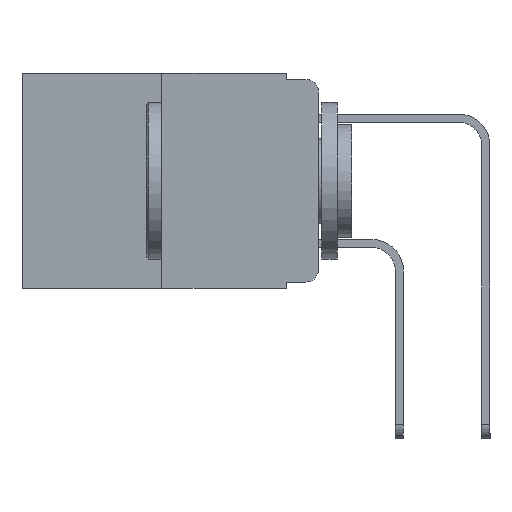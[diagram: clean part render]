
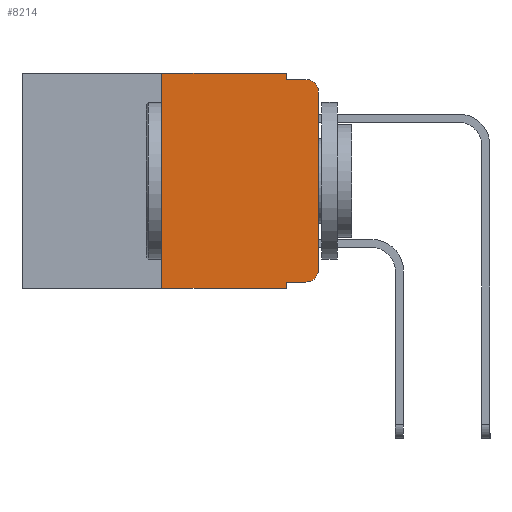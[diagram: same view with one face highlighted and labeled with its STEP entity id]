
A CAD part, left-side view. The second image highlights one B-rep face of the part: STEP entity #8214.
In plain terms, the highlighted planar face has unit normal (-1, 0, 0).
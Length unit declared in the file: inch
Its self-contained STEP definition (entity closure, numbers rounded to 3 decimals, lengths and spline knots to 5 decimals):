
#141 = CARTESIAN_POINT ( 'NONE',  ( 0., 0.473, -0.343 ) ) ;
#411 = EDGE_CURVE ( 'NONE', #4184, #6890, #11350, .T. ) ;
#431 = CARTESIAN_POINT ( 'NONE',  ( 0., 0.051, -0.333 ) ) ;
#1786 = CARTESIAN_POINT ( 'NONE',  ( 0., 0.25, 0. ) ) ;
#2180 = CARTESIAN_POINT ( 'NONE',  ( 0., 0.02, -0.333 ) ) ;
#2209 = DIRECTION ( 'NONE',  ( 0., -1., 0. ) ) ;
#2853 = AXIS2_PLACEMENT_3D ( 'NONE', #21239, #9372, #23160 ) ;
#2871 = CARTESIAN_POINT ( 'NONE',  ( 0., 0., -0.313 ) ) ;
#2944 = DIRECTION ( 'NONE',  ( 0., -1., 0. ) ) ;
#3098 = VERTEX_POINT ( 'NONE', #431 ) ;
#3100 = CARTESIAN_POINT ( 'NONE',  ( 0., 0.25, 0. ) ) ;
#3232 = VECTOR ( 'NONE', #19930, 39.37008 ) ;
#3301 = LINE ( 'NONE', #141, #13367 ) ;
#3305 = CARTESIAN_POINT ( 'NONE',  ( 0., 0.051, -0.343 ) ) ;
#3547 = CARTESIAN_POINT ( 'NONE',  ( 0., 0., -0.03 ) ) ;
#3550 = LINE ( 'NONE', #17707, #18863 ) ;
#3804 = DIRECTION ( 'NONE',  ( 0., 0., 1. ) ) ;
#4184 = VERTEX_POINT ( 'NONE', #2180 ) ;
#4240 = CARTESIAN_POINT ( 'NONE',  ( 0., 0.051, 0. ) ) ;
#4698 = EDGE_CURVE ( 'NONE', #12145, #19349, #23422, .T. ) ;
#4979 = PLANE ( 'NONE',  #25516 ) ;
#5031 = EDGE_CURVE ( 'NONE', #21617, #6190, #22497, .T. ) ;
#5187 = EDGE_CURVE ( 'NONE', #3098, #4184, #3550, .T. ) ;
#6190 = VERTEX_POINT ( 'NONE', #18696 ) ;
#6381 = EDGE_CURVE ( 'NONE', #14464, #6190, #7795, .T. ) ;
#6716 = VECTOR ( 'NONE', #2944, 39.37008 ) ;
#6890 = VERTEX_POINT ( 'NONE', #2871 ) ;
#6992 = DIRECTION ( 'NONE',  ( 0., 0., -1. ) ) ;
#7072 = FACE_OUTER_BOUND ( 'NONE', #13237, .T. ) ;
#7083 = VECTOR ( 'NONE', #19625, 39.37008 ) ;
#7795 = CIRCLE ( 'NONE', #2853, 0.02 ) ;
#8214 = ADVANCED_FACE ( 'NONE', ( #7072 ), #4979, .F. ) ;
#9088 = EDGE_CURVE ( 'NONE', #12145, #10170, #3301, .T. ) ;
#9372 = DIRECTION ( 'NONE',  ( -1., 0., 0. ) ) ;
#10170 = VERTEX_POINT ( 'NONE', #3305 ) ;
#10204 = ORIENTED_EDGE ( 'NONE', *, *, #9088, .T. ) ;
#10403 = EDGE_CURVE ( 'NONE', #6890, #14464, #13903, .T. ) ;
#11150 = AXIS2_PLACEMENT_3D ( 'NONE', #21232, #23412, #23553 ) ;
#11350 = CIRCLE ( 'NONE', #11150, 0.02 ) ;
#12002 = EDGE_CURVE ( 'NONE', #19349, #13975, #20592, .T. ) ;
#12145 = VERTEX_POINT ( 'NONE', #16692 ) ;
#12557 = ORIENTED_EDGE ( 'NONE', *, *, #10403, .T. ) ;
#13041 = VECTOR ( 'NONE', #3804, 39.37008 ) ;
#13237 = EDGE_LOOP ( 'NONE', ( #12557, #23017, #16154, #21878, #24249, #14866, #10204, #18603, #24890, #20110 ) ) ;
#13367 = VECTOR ( 'NONE', #2209, 39.37008 ) ;
#13903 = LINE ( 'NONE', #17967, #3232 ) ;
#13975 = VERTEX_POINT ( 'NONE', #20561 ) ;
#14464 = VERTEX_POINT ( 'NONE', #3547 ) ;
#14735 = VECTOR ( 'NONE', #22157, 39.37008 ) ;
#14866 = ORIENTED_EDGE ( 'NONE', *, *, #4698, .F. ) ;
#14943 = CARTESIAN_POINT ( 'NONE',  ( 0., 0.473, 0. ) ) ;
#16154 = ORIENTED_EDGE ( 'NONE', *, *, #5031, .F. ) ;
#16692 = CARTESIAN_POINT ( 'NONE',  ( 0., 0.25, -0.343 ) ) ;
#17244 = EDGE_CURVE ( 'NONE', #3098, #10170, #19143, .T. ) ;
#17673 = CARTESIAN_POINT ( 'NONE',  ( 0., 0.051, 0. ) ) ;
#17707 = CARTESIAN_POINT ( 'NONE',  ( 0., 0.051, -0.333 ) ) ;
#17967 = CARTESIAN_POINT ( 'NONE',  ( 0., 0., 0. ) ) ;
#18603 = ORIENTED_EDGE ( 'NONE', *, *, #17244, .F. ) ;
#18696 = CARTESIAN_POINT ( 'NONE',  ( 0., 0.02, -0.01 ) ) ;
#18863 = VECTOR ( 'NONE', #19659, 39.37008 ) ;
#18927 = DIRECTION ( 'NONE',  ( 1., 0., 0. ) ) ;
#19143 = LINE ( 'NONE', #4240, #23657 ) ;
#19349 = VERTEX_POINT ( 'NONE', #3100 ) ;
#19625 = DIRECTION ( 'NONE',  ( 0., 0., -1. ) ) ;
#19659 = DIRECTION ( 'NONE',  ( 0., -1., 0. ) ) ;
#19930 = DIRECTION ( 'NONE',  ( 0., 0., 1. ) ) ;
#19966 = CARTESIAN_POINT ( 'NONE',  ( 0., 0.051, -0.01 ) ) ;
#20110 = ORIENTED_EDGE ( 'NONE', *, *, #411, .T. ) ;
#20132 = CARTESIAN_POINT ( 'NONE',  ( 0., 0.473, 0. ) ) ;
#20172 = DIRECTION ( 'NONE',  ( 0., 0., -1. ) ) ;
#20561 = CARTESIAN_POINT ( 'NONE',  ( 0., 0.051, 0. ) ) ;
#20592 = LINE ( 'NONE', #20132, #14735 ) ;
#21232 = CARTESIAN_POINT ( 'NONE',  ( 0., 0.02, -0.313 ) ) ;
#21239 = CARTESIAN_POINT ( 'NONE',  ( 0., 0.02, -0.03 ) ) ;
#21491 = EDGE_CURVE ( 'NONE', #13975, #21617, #22856, .T. ) ;
#21617 = VERTEX_POINT ( 'NONE', #19966 ) ;
#21878 = ORIENTED_EDGE ( 'NONE', *, *, #21491, .F. ) ;
#22157 = DIRECTION ( 'NONE',  ( 0., -1., 0. ) ) ;
#22497 = LINE ( 'NONE', #24539, #6716 ) ;
#22856 = LINE ( 'NONE', #17673, #7083 ) ;
#23017 = ORIENTED_EDGE ( 'NONE', *, *, #6381, .T. ) ;
#23160 = DIRECTION ( 'NONE',  ( 0., 0., -1. ) ) ;
#23412 = DIRECTION ( 'NONE',  ( -1., 0., 0. ) ) ;
#23422 = LINE ( 'NONE', #1786, #13041 ) ;
#23553 = DIRECTION ( 'NONE',  ( 0., 0., -1. ) ) ;
#23657 = VECTOR ( 'NONE', #20172, 39.37008 ) ;
#24249 = ORIENTED_EDGE ( 'NONE', *, *, #12002, .F. ) ;
#24539 = CARTESIAN_POINT ( 'NONE',  ( 0., 0.051, -0.01 ) ) ;
#24890 = ORIENTED_EDGE ( 'NONE', *, *, #5187, .T. ) ;
#25516 = AXIS2_PLACEMENT_3D ( 'NONE', #14943, #18927, #6992 ) ;
